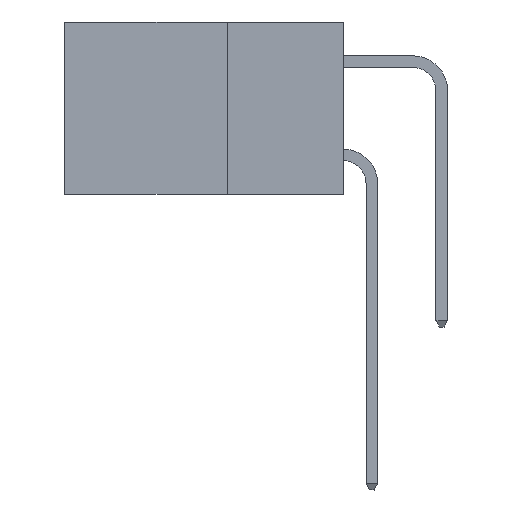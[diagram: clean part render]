
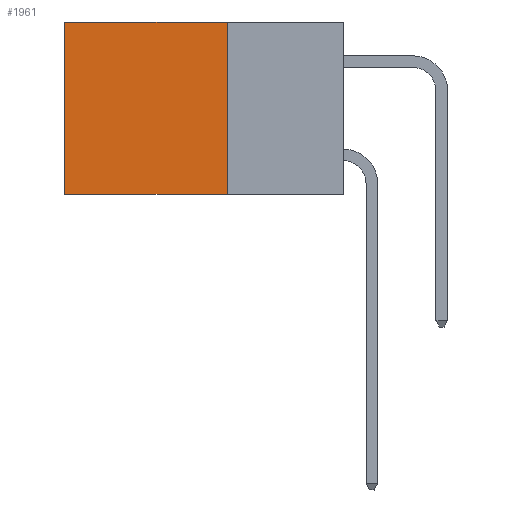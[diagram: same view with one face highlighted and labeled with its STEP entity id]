
A CAD part, left-side view. The second image highlights one B-rep face of the part: STEP entity #1961.
In plain terms, the highlighted planar face has unit normal (-1, 0, 0).
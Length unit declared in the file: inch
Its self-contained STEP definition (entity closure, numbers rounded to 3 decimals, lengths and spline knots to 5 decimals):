
#110 = ORIENTED_EDGE ( 'NONE', *, *, #13809, .T. ) ;
#467 = DIRECTION ( 'NONE',  ( 0., 0., -1. ) ) ;
#1172 = CARTESIAN_POINT ( 'NONE',  ( 0.2615, 0.25, 0. ) ) ;
#1864 = CARTESIAN_POINT ( 'NONE',  ( 0.2615, 0.25, -0.37 ) ) ;
#1961 = ADVANCED_FACE ( 'NONE', ( #7134 ), #8476, .F. ) ;
#2481 = VECTOR ( 'NONE', #10050, 39.37008 ) ;
#3113 = DIRECTION ( 'NONE',  ( 0., 0., -1. ) ) ;
#3639 = VERTEX_POINT ( 'NONE', #5690 ) ;
#3741 = DIRECTION ( 'NONE',  ( 0., 0., -1. ) ) ;
#3941 = CARTESIAN_POINT ( 'NONE',  ( 0.2615, 0.25, -0.37 ) ) ;
#4237 = LINE ( 'NONE', #1864, #7178 ) ;
#4306 = ORIENTED_EDGE ( 'NONE', *, *, #10261, .T. ) ;
#4565 = LINE ( 'NONE', #11215, #4615 ) ;
#4615 = VECTOR ( 'NONE', #5609, 39.37008 ) ;
#5136 = ORIENTED_EDGE ( 'NONE', *, *, #9632, .F. ) ;
#5267 = AXIS2_PLACEMENT_3D ( 'NONE', #13937, #11580, #3741 ) ;
#5609 = DIRECTION ( 'NONE',  ( 0., 1., 0. ) ) ;
#5690 = CARTESIAN_POINT ( 'NONE',  ( 0.2615, 0.6, 0. ) ) ;
#5832 = CARTESIAN_POINT ( 'NONE',  ( 0.2615, 0.25, 0. ) ) ;
#6990 = VERTEX_POINT ( 'NONE', #7484 ) ;
#7134 = FACE_OUTER_BOUND ( 'NONE', #13747, .T. ) ;
#7178 = VECTOR ( 'NONE', #3113, 39.37008 ) ;
#7484 = CARTESIAN_POINT ( 'NONE',  ( 0.2615, 0.6, -0.37 ) ) ;
#7784 = ORIENTED_EDGE ( 'NONE', *, *, #12055, .F. ) ;
#8351 = VERTEX_POINT ( 'NONE', #3941 ) ;
#8476 = PLANE ( 'NONE',  #5267 ) ;
#9016 = VERTEX_POINT ( 'NONE', #5832 ) ;
#9632 = EDGE_CURVE ( 'NONE', #9016, #8351, #4237, .T. ) ;
#10050 = DIRECTION ( 'NONE',  ( 0., 1., 0. ) ) ;
#10261 = EDGE_CURVE ( 'NONE', #9016, #3639, #13595, .T. ) ;
#10307 = VECTOR ( 'NONE', #467, 39.37008 ) ;
#10814 = CARTESIAN_POINT ( 'NONE',  ( 0.2615, 0.6, -0.37 ) ) ;
#11215 = CARTESIAN_POINT ( 'NONE',  ( 0.2615, 0.25, -0.37 ) ) ;
#11580 = DIRECTION ( 'NONE',  ( 1., 0., 0. ) ) ;
#12055 = EDGE_CURVE ( 'NONE', #8351, #6990, #4565, .T. ) ;
#13595 = LINE ( 'NONE', #1172, #2481 ) ;
#13702 = LINE ( 'NONE', #10814, #10307 ) ;
#13747 = EDGE_LOOP ( 'NONE', ( #110, #7784, #5136, #4306 ) ) ;
#13809 = EDGE_CURVE ( 'NONE', #3639, #6990, #13702, .T. ) ;
#13937 = CARTESIAN_POINT ( 'NONE',  ( 0.2615, 0.25, -0.37 ) ) ;
